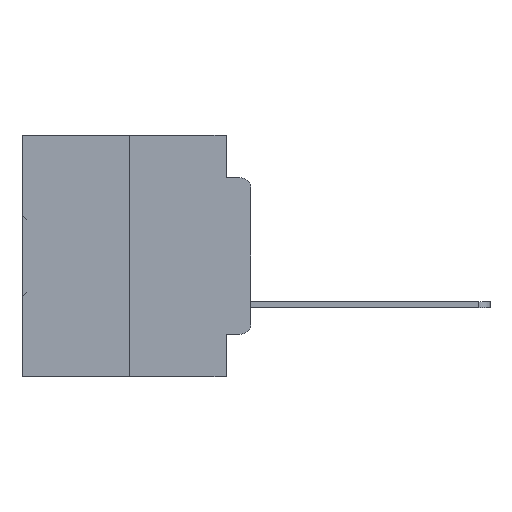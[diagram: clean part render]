
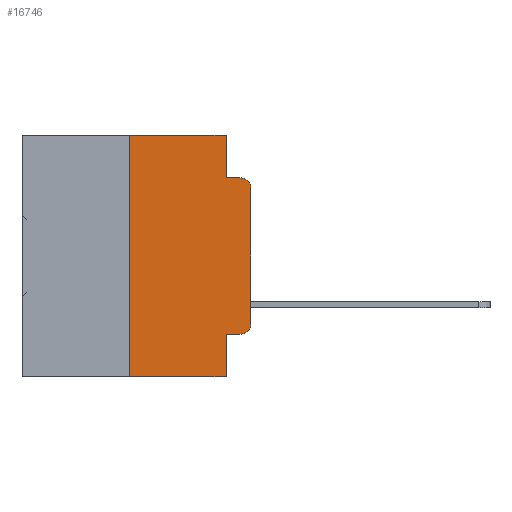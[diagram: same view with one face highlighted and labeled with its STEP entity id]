
A CAD part, left-side view. The second image highlights one B-rep face of the part: STEP entity #16746.
In plain terms, the highlighted planar face has unit normal (-1, 0, 0).
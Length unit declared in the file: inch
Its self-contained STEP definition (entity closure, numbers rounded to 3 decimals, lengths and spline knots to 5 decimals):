
#88 = VERTEX_POINT ( 'NONE', #22870 ) ;
#425 = ORIENTED_EDGE ( 'NONE', *, *, #19138, .T. ) ;
#588 = VERTEX_POINT ( 'NONE', #9629 ) ;
#768 = DIRECTION ( 'NONE',  ( 1., 0., 0. ) ) ;
#904 = VERTEX_POINT ( 'NONE', #24636 ) ;
#1113 = CARTESIAN_POINT ( 'NONE',  ( 0., 0.051, -0.0885 ) ) ;
#1286 = VERTEX_POINT ( 'NONE', #18699 ) ;
#1450 = EDGE_CURVE ( 'NONE', #4670, #33378, #3769, .T. ) ;
#1503 = EDGE_CURVE ( 'NONE', #588, #4670, #16941, .T. ) ;
#1727 = CARTESIAN_POINT ( 'NONE',  ( 0., 0., -0.3915 ) ) ;
#2100 = CARTESIAN_POINT ( 'NONE',  ( 0., 0.02, -0.0885 ) ) ;
#3398 = EDGE_CURVE ( 'NONE', #33378, #14186, #14220, .T. ) ;
#3769 = LINE ( 'NONE', #29848, #17803 ) ;
#4172 = LINE ( 'NONE', #7278, #26250 ) ;
#4351 = CARTESIAN_POINT ( 'NONE',  ( 0., 0.02, -0.1085 ) ) ;
#4670 = VERTEX_POINT ( 'NONE', #12768 ) ;
#4715 = CARTESIAN_POINT ( 'NONE',  ( 0., 0.02, -0.3915 ) ) ;
#4852 = ORIENTED_EDGE ( 'NONE', *, *, #5297, .T. ) ;
#5297 = EDGE_CURVE ( 'NONE', #1286, #14186, #18484, .T. ) ;
#6730 = CARTESIAN_POINT ( 'NONE',  ( 0., 0., 0. ) ) ;
#7228 = DIRECTION ( 'NONE',  ( 0., 0., -1. ) ) ;
#7278 = CARTESIAN_POINT ( 'NONE',  ( 0., 0.051, 0. ) ) ;
#7530 = ORIENTED_EDGE ( 'NONE', *, *, #1450, .F. ) ;
#7582 = DIRECTION ( 'NONE',  ( 0., 0., -1. ) ) ;
#7839 = AXIS2_PLACEMENT_3D ( 'NONE', #4351, #23778, #7228 ) ;
#9251 = CARTESIAN_POINT ( 'NONE',  ( 0., 0.473, 0. ) ) ;
#9629 = CARTESIAN_POINT ( 'NONE',  ( 0., 0.25, 0. ) ) ;
#9882 = DIRECTION ( 'NONE',  ( 0., -1., 0. ) ) ;
#10354 = VERTEX_POINT ( 'NONE', #13656 ) ;
#10403 = VECTOR ( 'NONE', #16755, 39.37008 ) ;
#11131 = CARTESIAN_POINT ( 'NONE',  ( 0., 0.473, 0. ) ) ;
#12768 = CARTESIAN_POINT ( 'NONE',  ( 0., 0.051, 0. ) ) ;
#12824 = EDGE_CURVE ( 'NONE', #17005, #1286, #13596, .T. ) ;
#12884 = DIRECTION ( 'NONE',  ( 0., 0., -1. ) ) ;
#13359 = VECTOR ( 'NONE', #17959, 39.37008 ) ;
#13596 = LINE ( 'NONE', #6730, #34335 ) ;
#13656 = CARTESIAN_POINT ( 'NONE',  ( 0., 0.02, -0.4115 ) ) ;
#14051 = ORIENTED_EDGE ( 'NONE', *, *, #3398, .F. ) ;
#14186 = VERTEX_POINT ( 'NONE', #2100 ) ;
#14220 = LINE ( 'NONE', #1113, #13359 ) ;
#14790 = VECTOR ( 'NONE', #9882, 39.37008 ) ;
#14825 = VERTEX_POINT ( 'NONE', #34932 ) ;
#15055 = DIRECTION ( 'NONE',  ( 0., -1., 0. ) ) ;
#15130 = DIRECTION ( 'NONE',  ( 0., 0., 1. ) ) ;
#15131 = DIRECTION ( 'NONE',  ( 0., 0., 1. ) ) ;
#16345 = CARTESIAN_POINT ( 'NONE',  ( 0., 0.051, -0.0885 ) ) ;
#16352 = EDGE_CURVE ( 'NONE', #14825, #904, #25909, .T. ) ;
#16709 = ORIENTED_EDGE ( 'NONE', *, *, #1503, .F. ) ;
#16746 = ADVANCED_FACE ( 'NONE', ( #20423 ), #30944, .F. ) ;
#16755 = DIRECTION ( 'NONE',  ( 0., -1., 0. ) ) ;
#16941 = LINE ( 'NONE', #11131, #10403 ) ;
#17005 = VERTEX_POINT ( 'NONE', #1727 ) ;
#17803 = VECTOR ( 'NONE', #24720, 39.37008 ) ;
#17959 = DIRECTION ( 'NONE',  ( 0., -1., 0. ) ) ;
#18484 = CIRCLE ( 'NONE', #7839, 0.02 ) ;
#18699 = CARTESIAN_POINT ( 'NONE',  ( 0., 0., -0.1085 ) ) ;
#18712 = VECTOR ( 'NONE', #15055, 39.37008 ) ;
#19138 = EDGE_CURVE ( 'NONE', #10354, #17005, #30273, .T. ) ;
#19983 = VECTOR ( 'NONE', #15131, 39.37008 ) ;
#20423 = FACE_OUTER_BOUND ( 'NONE', #20751, .T. ) ;
#20425 = DIRECTION ( 'NONE',  ( 0., 0., -1. ) ) ;
#20751 = EDGE_LOOP ( 'NONE', ( #33127, #4852, #14051, #7530, #16709, #26476, #33552, #34375, #28570, #425 ) ) ;
#20962 = EDGE_CURVE ( 'NONE', #88, #10354, #34642, .T. ) ;
#22756 = EDGE_CURVE ( 'NONE', #88, #904, #4172, .T. ) ;
#22870 = CARTESIAN_POINT ( 'NONE',  ( 0., 0.051, -0.4115 ) ) ;
#23301 = CARTESIAN_POINT ( 'NONE',  ( 0., 0.25, 0. ) ) ;
#23609 = CARTESIAN_POINT ( 'NONE',  ( 0., 0.051, -0.4115 ) ) ;
#23778 = DIRECTION ( 'NONE',  ( -1., 0., 0. ) ) ;
#24107 = DIRECTION ( 'NONE',  ( -1., 0., 0. ) ) ;
#24550 = EDGE_CURVE ( 'NONE', #14825, #588, #26289, .T. ) ;
#24636 = CARTESIAN_POINT ( 'NONE',  ( 0., 0.051, -0.5 ) ) ;
#24720 = DIRECTION ( 'NONE',  ( 0., 0., -1. ) ) ;
#25909 = LINE ( 'NONE', #33958, #18712 ) ;
#26250 = VECTOR ( 'NONE', #12884, 39.37008 ) ;
#26289 = LINE ( 'NONE', #23301, #19983 ) ;
#26476 = ORIENTED_EDGE ( 'NONE', *, *, #24550, .F. ) ;
#28570 = ORIENTED_EDGE ( 'NONE', *, *, #20962, .T. ) ;
#29848 = CARTESIAN_POINT ( 'NONE',  ( 0., 0.051, 0. ) ) ;
#30036 = AXIS2_PLACEMENT_3D ( 'NONE', #9251, #768, #20425 ) ;
#30273 = CIRCLE ( 'NONE', #33641, 0.02 ) ;
#30944 = PLANE ( 'NONE',  #30036 ) ;
#33127 = ORIENTED_EDGE ( 'NONE', *, *, #12824, .T. ) ;
#33378 = VERTEX_POINT ( 'NONE', #16345 ) ;
#33552 = ORIENTED_EDGE ( 'NONE', *, *, #16352, .T. ) ;
#33641 = AXIS2_PLACEMENT_3D ( 'NONE', #4715, #24107, #7582 ) ;
#33958 = CARTESIAN_POINT ( 'NONE',  ( 0., 0.473, -0.5 ) ) ;
#34335 = VECTOR ( 'NONE', #15130, 39.37008 ) ;
#34375 = ORIENTED_EDGE ( 'NONE', *, *, #22756, .F. ) ;
#34642 = LINE ( 'NONE', #23609, #14790 ) ;
#34932 = CARTESIAN_POINT ( 'NONE',  ( 0., 0.25, -0.5 ) ) ;
